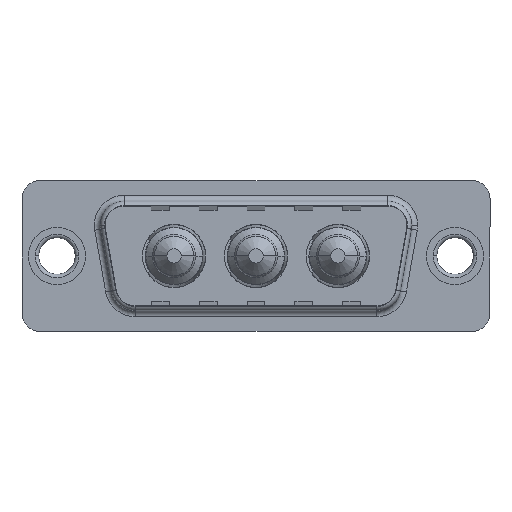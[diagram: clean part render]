
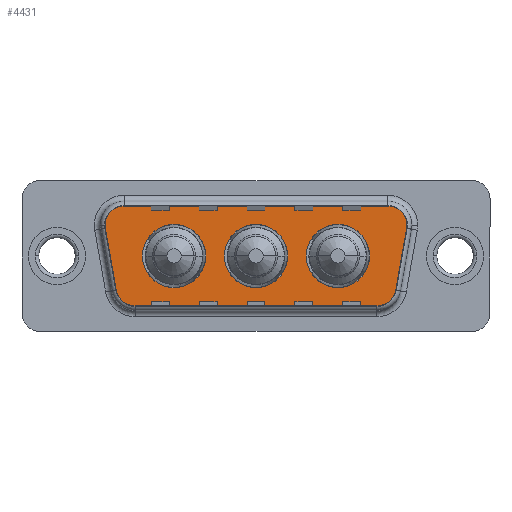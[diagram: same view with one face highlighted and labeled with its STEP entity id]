
A CAD part, top view. The second image highlights one B-rep face of the part: STEP entity #4431.
In plain terms, the highlighted planar face has unit normal (0, 0, 1).
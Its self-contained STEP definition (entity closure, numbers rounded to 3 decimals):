
#8 = CARTESIAN_POINT ( 'NONE',  ( 23.5, 0., 0. ) ) ;
#48 = CIRCLE ( 'NONE', #2279, 2.65 ) ;
#50 = DIRECTION ( 'NONE',  ( 0.174, -0.985, 0. ) ) ;
#221 = DIRECTION ( 'NONE',  ( 1., 0., 0. ) ) ;
#231 = AXIS2_PLACEMENT_3D ( 'NONE', #6747, #1499, #7610 ) ;
#256 = DIRECTION ( 'NONE',  ( 1., 0., 0. ) ) ;
#336 = CARTESIAN_POINT ( 'NONE',  ( 29.889, 2.9, 0. ) ) ;
#522 = ORIENTED_EDGE ( 'NONE', *, *, #2453, .T. ) ;
#665 = VERTEX_POINT ( 'NONE', #726 ) ;
#726 = CARTESIAN_POINT ( 'NONE',  ( 14., 0., 0. ) ) ;
#806 = VERTEX_POINT ( 'NONE', #4558 ) ;
#868 = FACE_BOUND ( 'NONE', #9659, .T. ) ;
#906 = EDGE_CURVE ( 'NONE', #3323, #7291, #5138, .T. ) ;
#919 = CARTESIAN_POINT ( 'NONE',  ( 5.411, 2.9, 0. ) ) ;
#1022 = DIRECTION ( 'NONE',  ( 0., 0., 1. ) ) ;
#1094 = AXIS2_PLACEMENT_3D ( 'NONE', #3920, #4942, #221 ) ;
#1137 = FACE_BOUND ( 'NONE', #10309, .T. ) ;
#1165 = PLANE ( 'NONE',  #7141 ) ;
#1209 = CARTESIAN_POINT ( 'NONE',  ( 16.65, 0., 0. ) ) ;
#1322 = AXIS2_PLACEMENT_3D ( 'NONE', #1632, #7747, #2480 ) ;
#1483 = EDGE_CURVE ( 'NONE', #4398, #2838, #48, .T. ) ;
#1499 = DIRECTION ( 'NONE',  ( 0., 0., 1. ) ) ;
#1516 = VERTEX_POINT ( 'NONE', #5271 ) ;
#1614 = DIRECTION ( 'NONE',  ( 0., 0., 1. ) ) ;
#1632 = CARTESIAN_POINT ( 'NONE',  ( 16.65, 0., 0. ) ) ;
#1762 = CARTESIAN_POINT ( 'NONE',  ( 9.8, 0., 0. ) ) ;
#1819 = CIRCLE ( 'NONE', #7975, 2.65 ) ;
#2008 = DIRECTION ( 'NONE',  ( -1., 0., 0. ) ) ;
#2068 = CARTESIAN_POINT ( 'NONE',  ( 6.434, -4.9, 0. ) ) ;
#2174 = EDGE_LOOP ( 'NONE', ( #6204, #8173, #2763, #522, #8415, #10969, #6260, #6789, #6321 ) ) ;
#2175 = ORIENTED_EDGE ( 'NONE', *, *, #3619, .F. ) ;
#2222 = CARTESIAN_POINT ( 'NONE',  ( 7.15, 0., 0. ) ) ;
#2279 = AXIS2_PLACEMENT_3D ( 'NONE', #6740, #6731, #4867 ) ;
#2328 = EDGE_CURVE ( 'NONE', #10364, #1516, #5813, .T. ) ;
#2408 = EDGE_CURVE ( 'NONE', #8637, #8635, #6522, .T. ) ;
#2453 = EDGE_CURVE ( 'NONE', #7014, #6993, #6240, .T. ) ;
#2480 = DIRECTION ( 'NONE',  ( 1., 0., 0. ) ) ;
#2763 = ORIENTED_EDGE ( 'NONE', *, *, #10673, .T. ) ;
#2838 = VERTEX_POINT ( 'NONE', #2222 ) ;
#2944 = DIRECTION ( 'NONE',  ( 0., 0., 1. ) ) ;
#2991 = EDGE_CURVE ( 'NONE', #8635, #3323, #4554, .T. ) ;
#3069 = DIRECTION ( 'NONE',  ( 0., 0., 1. ) ) ;
#3133 = CARTESIAN_POINT ( 'NONE',  ( 12.45, 0., 0. ) ) ;
#3139 = FACE_OUTER_BOUND ( 'NONE', #2174, .T. ) ;
#3233 = AXIS2_PLACEMENT_3D ( 'NONE', #919, #3621, #256 ) ;
#3323 = VERTEX_POINT ( 'NONE', #2068 ) ;
#3614 = EDGE_CURVE ( 'NONE', #1516, #10364, #1819, .T. ) ;
#3619 = EDGE_CURVE ( 'NONE', #665, #4939, #6751, .T. ) ;
#3621 = DIRECTION ( 'NONE',  ( 0., 0., 1. ) ) ;
#3628 = EDGE_LOOP ( 'NONE', ( #6470, #2175 ) ) ;
#3736 = AXIS2_PLACEMENT_3D ( 'NONE', #9689, #1022, #9884 ) ;
#3920 = CARTESIAN_POINT ( 'NONE',  ( 26.866, -2.9, 0. ) ) ;
#4147 = CARTESIAN_POINT ( 'NONE',  ( 6.434, -4.9, 0. ) ) ;
#4151 = VECTOR ( 'NONE', #50, 1000. ) ;
#4183 = CARTESIAN_POINT ( 'NONE',  ( 3.441, 2.553, 0. ) ) ;
#4283 = CARTESIAN_POINT ( 'NONE',  ( 5.411, 4.9, 0. ) ) ;
#4305 = VERTEX_POINT ( 'NONE', #5947 ) ;
#4398 = VERTEX_POINT ( 'NONE', #3133 ) ;
#4431 = ADVANCED_FACE ( 'NONE', ( #5477, #868, #1137, #3139 ), #1165, .T. ) ;
#4515 = DIRECTION ( 'NONE',  ( 1., 0., 0. ) ) ;
#4554 = CIRCLE ( 'NONE', #5126, 2. ) ;
#4558 = CARTESIAN_POINT ( 'NONE',  ( 29.859, 2.553, 0. ) ) ;
#4606 = CARTESIAN_POINT ( 'NONE',  ( 29.859, 2.553, 0. ) ) ;
#4649 = CARTESIAN_POINT ( 'NONE',  ( 23.5, 0., 0. ) ) ;
#4711 = DIRECTION ( 'NONE',  ( 1., 0., 0. ) ) ;
#4867 = DIRECTION ( 'NONE',  ( 1., 0., 0. ) ) ;
#4939 = VERTEX_POINT ( 'NONE', #9584 ) ;
#4942 = DIRECTION ( 'NONE',  ( 0., 0., 1. ) ) ;
#5076 = CARTESIAN_POINT ( 'NONE',  ( 26.866, -4.9, 0. ) ) ;
#5097 = CIRCLE ( 'NONE', #1094, 2. ) ;
#5126 = AXIS2_PLACEMENT_3D ( 'NONE', #7633, #9204, #2008 ) ;
#5138 = LINE ( 'NONE', #4147, #9712 ) ;
#5244 = ORIENTED_EDGE ( 'NONE', *, *, #5289, .F. ) ;
#5271 = CARTESIAN_POINT ( 'NONE',  ( 20.85, 0., 0. ) ) ;
#5289 = EDGE_CURVE ( 'NONE', #2838, #4398, #8556, .T. ) ;
#5313 = CIRCLE ( 'NONE', #231, 2. ) ;
#5477 = FACE_BOUND ( 'NONE', #3628, .T. ) ;
#5488 = DIRECTION ( 'NONE',  ( 0.174, 0.985, 0. ) ) ;
#5746 = DIRECTION ( 'NONE',  ( 1., 0., 0. ) ) ;
#5773 = LINE ( 'NONE', #4283, #10054 ) ;
#5803 = ORIENTED_EDGE ( 'NONE', *, *, #1483, .F. ) ;
#5813 = CIRCLE ( 'NONE', #6937, 2.65 ) ;
#5846 = LINE ( 'NONE', #4606, #10410 ) ;
#5934 = CARTESIAN_POINT ( 'NONE',  ( 28.836, -3.247, 0. ) ) ;
#5947 = CARTESIAN_POINT ( 'NONE',  ( 5.411, 4.9, 0. ) ) ;
#6111 = EDGE_CURVE ( 'NONE', #4305, #8637, #9420, .T. ) ;
#6204 = ORIENTED_EDGE ( 'NONE', *, *, #6672, .T. ) ;
#6240 = CIRCLE ( 'NONE', #3736, 2. ) ;
#6260 = ORIENTED_EDGE ( 'NONE', *, *, #2408, .T. ) ;
#6321 = ORIENTED_EDGE ( 'NONE', *, *, #906, .T. ) ;
#6470 = ORIENTED_EDGE ( 'NONE', *, *, #10763, .F. ) ;
#6522 = LINE ( 'NONE', #8749, #4151 ) ;
#6672 = EDGE_CURVE ( 'NONE', #7291, #8170, #5097, .T. ) ;
#6731 = DIRECTION ( 'NONE',  ( 0., 0., 1. ) ) ;
#6740 = CARTESIAN_POINT ( 'NONE',  ( 9.8, 0., 0. ) ) ;
#6747 = CARTESIAN_POINT ( 'NONE',  ( 27.889, 2.9, 0. ) ) ;
#6751 = CIRCLE ( 'NONE', #10249, 2.65 ) ;
#6789 = ORIENTED_EDGE ( 'NONE', *, *, #2991, .T. ) ;
#6793 = DIRECTION ( 'NONE',  ( 1., 0., 0. ) ) ;
#6842 = EDGE_CURVE ( 'NONE', #6993, #4305, #5773, .T. ) ;
#6937 = AXIS2_PLACEMENT_3D ( 'NONE', #4649, #3069, #4515 ) ;
#6993 = VERTEX_POINT ( 'NONE', #9251 ) ;
#7014 = VERTEX_POINT ( 'NONE', #336 ) ;
#7141 = AXIS2_PLACEMENT_3D ( 'NONE', #7901, #2944, #5746 ) ;
#7291 = VERTEX_POINT ( 'NONE', #5076 ) ;
#7295 = DIRECTION ( 'NONE',  ( 0., 0., 1. ) ) ;
#7610 = DIRECTION ( 'NONE',  ( -1., 0., 0. ) ) ;
#7633 = CARTESIAN_POINT ( 'NONE',  ( 6.434, -2.9, 0. ) ) ;
#7747 = DIRECTION ( 'NONE',  ( 0., 0., 1. ) ) ;
#7848 = DIRECTION ( 'NONE',  ( 1., 0., 0. ) ) ;
#7901 = CARTESIAN_POINT ( 'NONE',  ( 26.866, -2.9, 0. ) ) ;
#7975 = AXIS2_PLACEMENT_3D ( 'NONE', #8, #9488, #9883 ) ;
#8071 = ORIENTED_EDGE ( 'NONE', *, *, #2328, .F. ) ;
#8170 = VERTEX_POINT ( 'NONE', #5934 ) ;
#8173 = ORIENTED_EDGE ( 'NONE', *, *, #10931, .T. ) ;
#8402 = CARTESIAN_POINT ( 'NONE',  ( 4.464, -3.247, 0. ) ) ;
#8415 = ORIENTED_EDGE ( 'NONE', *, *, #6842, .T. ) ;
#8556 = CIRCLE ( 'NONE', #10264, 2.65 ) ;
#8635 = VERTEX_POINT ( 'NONE', #8402 ) ;
#8637 = VERTEX_POINT ( 'NONE', #4183 ) ;
#8749 = CARTESIAN_POINT ( 'NONE',  ( 3.441, 2.553, 0. ) ) ;
#8859 = CARTESIAN_POINT ( 'NONE',  ( 26.15, 0., 0. ) ) ;
#9204 = DIRECTION ( 'NONE',  ( 0., 0., 1. ) ) ;
#9251 = CARTESIAN_POINT ( 'NONE',  ( 27.889, 4.9, 0. ) ) ;
#9420 = CIRCLE ( 'NONE', #3233, 2. ) ;
#9488 = DIRECTION ( 'NONE',  ( 0., 0., 1. ) ) ;
#9584 = CARTESIAN_POINT ( 'NONE',  ( 19.3, 0., 0. ) ) ;
#9659 = EDGE_LOOP ( 'NONE', ( #8071, #11010 ) ) ;
#9689 = CARTESIAN_POINT ( 'NONE',  ( 27.889, 2.9, 0. ) ) ;
#9712 = VECTOR ( 'NONE', #4711, 1000. ) ;
#9883 = DIRECTION ( 'NONE',  ( 1., 0., 0. ) ) ;
#9884 = DIRECTION ( 'NONE',  ( -1., 0., 0. ) ) ;
#10054 = VECTOR ( 'NONE', #10632, 1000. ) ;
#10249 = AXIS2_PLACEMENT_3D ( 'NONE', #1209, #7295, #6793 ) ;
#10264 = AXIS2_PLACEMENT_3D ( 'NONE', #1762, #1614, #7848 ) ;
#10273 = CIRCLE ( 'NONE', #1322, 2.65 ) ;
#10309 = EDGE_LOOP ( 'NONE', ( #5803, #5244 ) ) ;
#10364 = VERTEX_POINT ( 'NONE', #8859 ) ;
#10410 = VECTOR ( 'NONE', #5488, 1000. ) ;
#10632 = DIRECTION ( 'NONE',  ( -1., 0., 0. ) ) ;
#10673 = EDGE_CURVE ( 'NONE', #806, #7014, #5313, .T. ) ;
#10763 = EDGE_CURVE ( 'NONE', #4939, #665, #10273, .T. ) ;
#10931 = EDGE_CURVE ( 'NONE', #8170, #806, #5846, .T. ) ;
#10969 = ORIENTED_EDGE ( 'NONE', *, *, #6111, .T. ) ;
#11010 = ORIENTED_EDGE ( 'NONE', *, *, #3614, .F. ) ;
